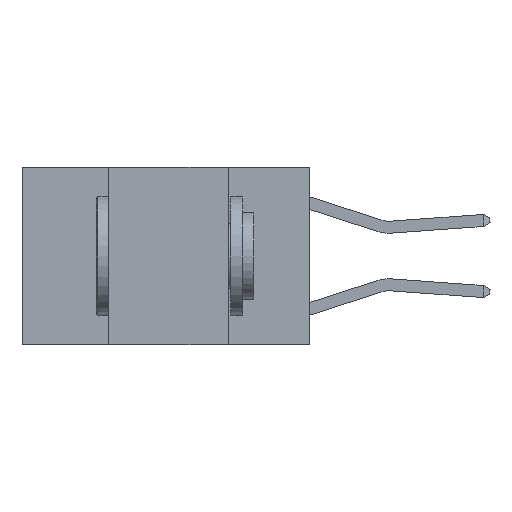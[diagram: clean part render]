
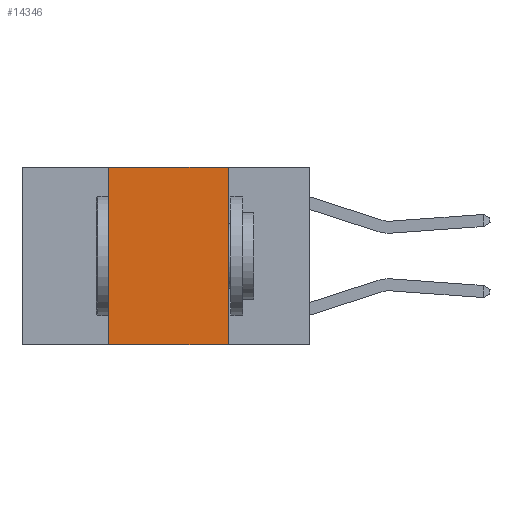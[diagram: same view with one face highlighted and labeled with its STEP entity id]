
A CAD part, left-side view. The second image highlights one B-rep face of the part: STEP entity #14346.
In plain terms, the highlighted planar face has unit normal (-1, 0, 0).
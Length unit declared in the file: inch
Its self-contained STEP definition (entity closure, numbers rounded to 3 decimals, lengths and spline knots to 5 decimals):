
#73 = FACE_OUTER_BOUND ( 'NONE', #7266, .T. ) ;
#720 = LINE ( 'NONE', #22979, #28065 ) ;
#735 = ORIENTED_EDGE ( 'NONE', *, *, #9901, .T. ) ;
#1039 = DIRECTION ( 'NONE',  ( 0., -1., 0. ) ) ;
#1205 = ORIENTED_EDGE ( 'NONE', *, *, #24104, .F. ) ;
#2351 = DIRECTION ( 'NONE',  ( 0., 0., -1. ) ) ;
#3356 = CARTESIAN_POINT ( 'NONE',  ( 0., 0.6, -0.37 ) ) ;
#5560 = VECTOR ( 'NONE', #6911, 39.37008 ) ;
#6911 = DIRECTION ( 'NONE',  ( 0., 0., -1. ) ) ;
#7266 = EDGE_LOOP ( 'NONE', ( #20872, #13602, #1205, #735 ) ) ;
#7423 = VERTEX_POINT ( 'NONE', #19542 ) ;
#8322 = EDGE_CURVE ( 'NONE', #15983, #30673, #19154, .T. ) ;
#9059 = CARTESIAN_POINT ( 'NONE',  ( 0., 0.42, 0. ) ) ;
#9452 = PLANE ( 'NONE',  #22357 ) ;
#9483 = CARTESIAN_POINT ( 'NONE',  ( 0., 0.17, 0. ) ) ;
#9901 = EDGE_CURVE ( 'NONE', #15756, #30673, #10432, .T. ) ;
#10432 = LINE ( 'NONE', #3356, #15022 ) ;
#10453 = CARTESIAN_POINT ( 'NONE',  ( 0., 0.42, -0.37 ) ) ;
#11479 = LINE ( 'NONE', #9059, #24292 ) ;
#13602 = ORIENTED_EDGE ( 'NONE', *, *, #29159, .F. ) ;
#14346 = ADVANCED_FACE ( 'NONE', ( #73 ), #9452, .F. ) ;
#15022 = VECTOR ( 'NONE', #30112, 39.37008 ) ;
#15756 = VERTEX_POINT ( 'NONE', #10453 ) ;
#15983 = VERTEX_POINT ( 'NONE', #17000 ) ;
#16865 = CARTESIAN_POINT ( 'NONE',  ( 0., 0.6, 0. ) ) ;
#17000 = CARTESIAN_POINT ( 'NONE',  ( 0., 0.17, 0. ) ) ;
#19154 = LINE ( 'NONE', #9483, #5560 ) ;
#19542 = CARTESIAN_POINT ( 'NONE',  ( 0., 0.42, 0. ) ) ;
#20872 = ORIENTED_EDGE ( 'NONE', *, *, #8322, .F. ) ;
#21302 = DIRECTION ( 'NONE',  ( 0., 0., 1. ) ) ;
#22357 = AXIS2_PLACEMENT_3D ( 'NONE', #16865, #29765, #2351 ) ;
#22979 = CARTESIAN_POINT ( 'NONE',  ( 0., 0.6, 0. ) ) ;
#23019 = CARTESIAN_POINT ( 'NONE',  ( 0., 0.17, -0.37 ) ) ;
#24104 = EDGE_CURVE ( 'NONE', #15756, #7423, #11479, .T. ) ;
#24292 = VECTOR ( 'NONE', #21302, 39.37008 ) ;
#28065 = VECTOR ( 'NONE', #1039, 39.37008 ) ;
#29159 = EDGE_CURVE ( 'NONE', #7423, #15983, #720, .T. ) ;
#29765 = DIRECTION ( 'NONE',  ( 1., 0., 0. ) ) ;
#30112 = DIRECTION ( 'NONE',  ( 0., -1., 0. ) ) ;
#30673 = VERTEX_POINT ( 'NONE', #23019 ) ;
